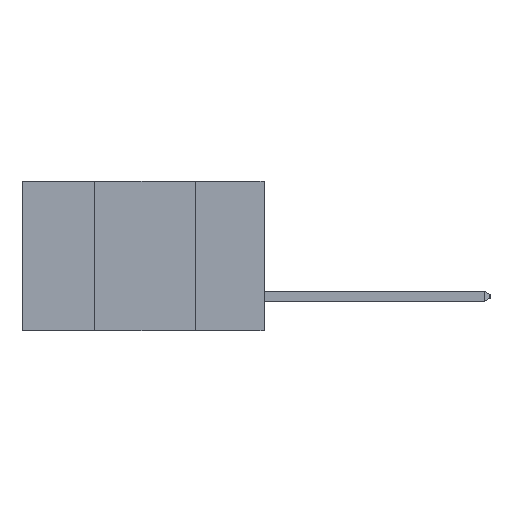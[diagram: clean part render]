
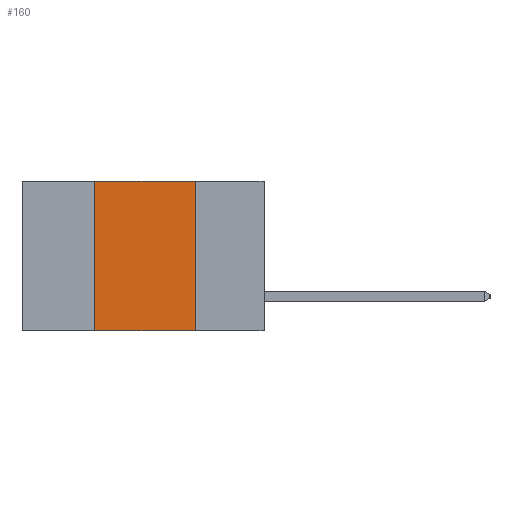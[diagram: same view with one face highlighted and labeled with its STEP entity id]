
A CAD part, left-side view. The second image highlights one B-rep face of the part: STEP entity #160.
In plain terms, the highlighted planar face has unit normal (-1, 0, 0).
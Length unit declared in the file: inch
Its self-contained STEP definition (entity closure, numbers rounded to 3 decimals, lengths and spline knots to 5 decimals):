
#160 = ADVANCED_FACE ( 'NONE', ( #18473 ), #8408, .F. ) ;
#1048 = AXIS2_PLACEMENT_3D ( 'NONE', #6057, #10776, #9155 ) ;
#2340 = CARTESIAN_POINT ( 'NONE',  ( 0., 0.17, -0.37 ) ) ;
#2639 = LINE ( 'NONE', #10122, #10822 ) ;
#2832 = VERTEX_POINT ( 'NONE', #17966 ) ;
#2885 = CARTESIAN_POINT ( 'NONE',  ( 0., 0.6, 0. ) ) ;
#4411 = DIRECTION ( 'NONE',  ( 0., -1., 0. ) ) ;
#4517 = CARTESIAN_POINT ( 'NONE',  ( 0., 0.17, 0. ) ) ;
#5677 = ORIENTED_EDGE ( 'NONE', *, *, #12150, .F. ) ;
#6057 = CARTESIAN_POINT ( 'NONE',  ( 0., 0.6, 0. ) ) ;
#6885 = CARTESIAN_POINT ( 'NONE',  ( 0., 0.17, -0.37 ) ) ;
#6950 = EDGE_LOOP ( 'NONE', ( #5677, #11664, #16855, #18061 ) ) ;
#7080 = VECTOR ( 'NONE', #4411, 39.37008 ) ;
#8408 = PLANE ( 'NONE',  #1048 ) ;
#8992 = EDGE_CURVE ( 'NONE', #2832, #12635, #2639, .T. ) ;
#9155 = DIRECTION ( 'NONE',  ( 0., 0., -1. ) ) ;
#9905 = LINE ( 'NONE', #2340, #14639 ) ;
#10010 = DIRECTION ( 'NONE',  ( 0., -1., 0. ) ) ;
#10031 = EDGE_CURVE ( 'NONE', #2832, #20035, #17688, .T. ) ;
#10122 = CARTESIAN_POINT ( 'NONE',  ( 0., 0.6, -0.37 ) ) ;
#10776 = DIRECTION ( 'NONE',  ( 1., 0., 0. ) ) ;
#10822 = VECTOR ( 'NONE', #10010, 39.37008 ) ;
#11107 = EDGE_CURVE ( 'NONE', #20035, #11709, #15427, .T. ) ;
#11664 = ORIENTED_EDGE ( 'NONE', *, *, #11107, .F. ) ;
#11709 = VERTEX_POINT ( 'NONE', #4517 ) ;
#12150 = EDGE_CURVE ( 'NONE', #11709, #12635, #9905, .T. ) ;
#12635 = VERTEX_POINT ( 'NONE', #6885 ) ;
#13473 = VECTOR ( 'NONE', #15669, 39.37008 ) ;
#14639 = VECTOR ( 'NONE', #14778, 39.37008 ) ;
#14778 = DIRECTION ( 'NONE',  ( 0., 0., -1. ) ) ;
#15427 = LINE ( 'NONE', #2885, #7080 ) ;
#15669 = DIRECTION ( 'NONE',  ( 0., 0., 1. ) ) ;
#15881 = CARTESIAN_POINT ( 'NONE',  ( 0., 0.42, -0.37 ) ) ;
#16855 = ORIENTED_EDGE ( 'NONE', *, *, #10031, .F. ) ;
#17688 = LINE ( 'NONE', #15881, #13473 ) ;
#17966 = CARTESIAN_POINT ( 'NONE',  ( 0., 0.42, -0.37 ) ) ;
#18061 = ORIENTED_EDGE ( 'NONE', *, *, #8992, .T. ) ;
#18473 = FACE_OUTER_BOUND ( 'NONE', #6950, .T. ) ;
#19286 = CARTESIAN_POINT ( 'NONE',  ( 0., 0.42, 0. ) ) ;
#20035 = VERTEX_POINT ( 'NONE', #19286 ) ;
